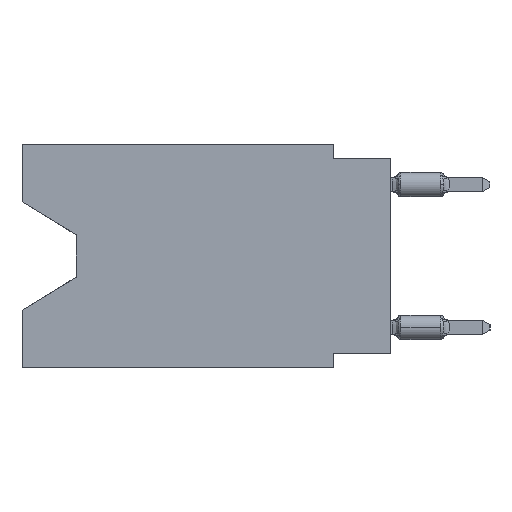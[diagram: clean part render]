
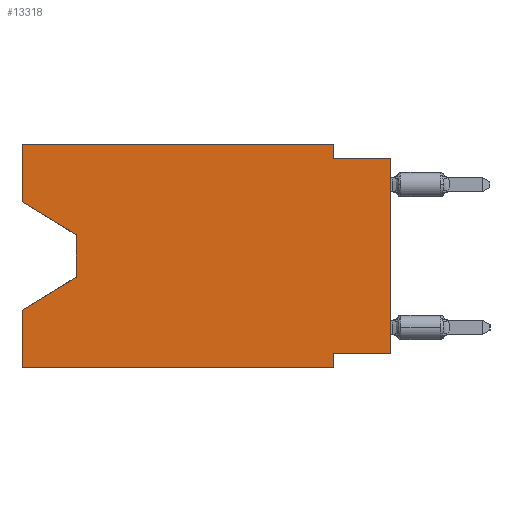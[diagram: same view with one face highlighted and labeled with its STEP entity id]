
A CAD part, left-side view. The second image highlights one B-rep face of the part: STEP entity #13318.
In plain terms, the highlighted planar face has unit normal (-1, 0, 0).
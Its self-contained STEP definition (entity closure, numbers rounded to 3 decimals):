
#568 = CARTESIAN_POINT ( 'NONE',  ( 0., 0., -9.271 ) ) ;
#723 = PLANE ( 'NONE',  #55464 ) ;
#1329 = VERTEX_POINT ( 'NONE', #13001 ) ;
#1730 = VERTEX_POINT ( 'NONE', #40131 ) ;
#1859 = DIRECTION ( 'NONE',  ( 0., 0.855, -0.519 ) ) ;
#2836 = VECTOR ( 'NONE', #10460, 1000. ) ;
#4807 = CARTESIAN_POINT ( 'NONE',  ( 0., 13.97, -5.893 ) ) ;
#6092 = DIRECTION ( 'NONE',  ( 0., 0., -1. ) ) ;
#6950 = LINE ( 'NONE', #62082, #31623 ) ;
#7746 = VERTEX_POINT ( 'NONE', #16965 ) ;
#8051 = VERTEX_POINT ( 'NONE', #4807 ) ;
#9061 = ORIENTED_EDGE ( 'NONE', *, *, #9385, .F. ) ;
#9385 = EDGE_CURVE ( 'NONE', #15146, #33059, #26433, .T. ) ;
#10120 = VERTEX_POINT ( 'NONE', #34221 ) ;
#10443 = EDGE_CURVE ( 'NONE', #60541, #45017, #34143, .T. ) ;
#10460 = DIRECTION ( 'NONE',  ( 0., 0., 1. ) ) ;
#10571 = EDGE_CURVE ( 'NONE', #13068, #45017, #55422, .T. ) ;
#11564 = ORIENTED_EDGE ( 'NONE', *, *, #10571, .T. ) ;
#13001 = CARTESIAN_POINT ( 'NONE',  ( 0., 16.383, 0. ) ) ;
#13068 = VERTEX_POINT ( 'NONE', #45047 ) ;
#13272 = EDGE_CURVE ( 'NONE', #7746, #8051, #41079, .T. ) ;
#13286 = ORIENTED_EDGE ( 'NONE', *, *, #41180, .T. ) ;
#13318 = ADVANCED_FACE ( 'NONE', ( #35832 ), #723, .F. ) ;
#14314 = VECTOR ( 'NONE', #6092, 1000. ) ;
#14420 = DIRECTION ( 'NONE',  ( 0., -1., 0. ) ) ;
#15146 = VERTEX_POINT ( 'NONE', #20239 ) ;
#16104 = EDGE_CURVE ( 'NONE', #53267, #1329, #44271, .T. ) ;
#16393 = DIRECTION ( 'NONE',  ( 0., -0.855, -0.519 ) ) ;
#16965 = CARTESIAN_POINT ( 'NONE',  ( 0., 13.97, -4.013 ) ) ;
#17095 = DIRECTION ( 'NONE',  ( 1., 0., 0. ) ) ;
#19294 = CARTESIAN_POINT ( 'NONE',  ( 0., 16.383, 0. ) ) ;
#19420 = CARTESIAN_POINT ( 'NONE',  ( 0., 2.54, -0.635 ) ) ;
#20239 = CARTESIAN_POINT ( 'NONE',  ( 0., 2.54, -9.271 ) ) ;
#20812 = EDGE_CURVE ( 'NONE', #1730, #60541, #23196, .T. ) ;
#20881 = LINE ( 'NONE', #568, #38752 ) ;
#20978 = VECTOR ( 'NONE', #16393, 1000. ) ;
#21396 = DIRECTION ( 'NONE',  ( 0., -1., 0. ) ) ;
#21693 = VECTOR ( 'NONE', #14420, 1000. ) ;
#23196 = LINE ( 'NONE', #32406, #49706 ) ;
#23734 = EDGE_CURVE ( 'NONE', #10120, #26596, #60609, .T. ) ;
#25001 = EDGE_CURVE ( 'NONE', #13068, #15146, #20881, .T. ) ;
#25100 = CARTESIAN_POINT ( 'NONE',  ( 0., 16.383, -9.906 ) ) ;
#26159 = ORIENTED_EDGE ( 'NONE', *, *, #42830, .F. ) ;
#26412 = EDGE_LOOP ( 'NONE', ( #13286, #37111, #46792, #61126, #58222, #9061, #44586, #11564, #39066, #61613, #26159, #39745 ) ) ;
#26433 = LINE ( 'NONE', #32013, #14314 ) ;
#26484 = CARTESIAN_POINT ( 'NONE',  ( 0., 16.383, -2.546 ) ) ;
#26596 = VERTEX_POINT ( 'NONE', #39900 ) ;
#29530 = VECTOR ( 'NONE', #35047, 1000. ) ;
#30913 = CARTESIAN_POINT ( 'NONE',  ( 0., 13.97, -4.013 ) ) ;
#31222 = DIRECTION ( 'NONE',  ( 0., 0., -1. ) ) ;
#31623 = VECTOR ( 'NONE', #21396, 1000. ) ;
#32001 = EDGE_CURVE ( 'NONE', #10120, #33059, #51000, .T. ) ;
#32013 = CARTESIAN_POINT ( 'NONE',  ( 0., 2.54, -9.906 ) ) ;
#32406 = CARTESIAN_POINT ( 'NONE',  ( 0., 2.54, 0. ) ) ;
#33059 = VERTEX_POINT ( 'NONE', #64493 ) ;
#33356 = LINE ( 'NONE', #53362, #51188 ) ;
#34143 = LINE ( 'NONE', #63008, #21693 ) ;
#34221 = CARTESIAN_POINT ( 'NONE',  ( 0., 16.383, -9.906 ) ) ;
#35047 = DIRECTION ( 'NONE',  ( 0., 0., 1. ) ) ;
#35345 = DIRECTION ( 'NONE',  ( 0., 0., 1. ) ) ;
#35832 = FACE_OUTER_BOUND ( 'NONE', #26412, .T. ) ;
#37111 = ORIENTED_EDGE ( 'NONE', *, *, #13272, .T. ) ;
#38304 = DIRECTION ( 'NONE',  ( 0., 0., -1. ) ) ;
#38752 = VECTOR ( 'NONE', #61895, 1000. ) ;
#39066 = ORIENTED_EDGE ( 'NONE', *, *, #10443, .F. ) ;
#39745 = ORIENTED_EDGE ( 'NONE', *, *, #16104, .F. ) ;
#39900 = CARTESIAN_POINT ( 'NONE',  ( 0., 16.383, -7.36 ) ) ;
#40131 = CARTESIAN_POINT ( 'NONE',  ( 0., 2.54, 0. ) ) ;
#40755 = DIRECTION ( 'NONE',  ( 0., 0., -1. ) ) ;
#41079 = LINE ( 'NONE', #30913, #46043 ) ;
#41180 = EDGE_CURVE ( 'NONE', #53267, #7746, #46616, .T. ) ;
#42830 = EDGE_CURVE ( 'NONE', #1329, #1730, #6950, .T. ) ;
#44271 = LINE ( 'NONE', #19294, #29530 ) ;
#44586 = ORIENTED_EDGE ( 'NONE', *, *, #25001, .F. ) ;
#45017 = VERTEX_POINT ( 'NONE', #62282 ) ;
#45047 = CARTESIAN_POINT ( 'NONE',  ( 0., 0., -9.271 ) ) ;
#45124 = DIRECTION ( 'NONE',  ( 0., -1., 0. ) ) ;
#45584 = CARTESIAN_POINT ( 'NONE',  ( 0., 0., 0. ) ) ;
#46043 = VECTOR ( 'NONE', #31222, 1000. ) ;
#46616 = LINE ( 'NONE', #56112, #20978 ) ;
#46792 = ORIENTED_EDGE ( 'NONE', *, *, #52120, .T. ) ;
#49706 = VECTOR ( 'NONE', #38304, 1000. ) ;
#51000 = LINE ( 'NONE', #25100, #62242 ) ;
#51188 = VECTOR ( 'NONE', #1859, 1000. ) ;
#52120 = EDGE_CURVE ( 'NONE', #8051, #26596, #33356, .T. ) ;
#53267 = VERTEX_POINT ( 'NONE', #26484 ) ;
#53362 = CARTESIAN_POINT ( 'NONE',  ( 0., 13.97, -5.893 ) ) ;
#55422 = LINE ( 'NONE', #45584, #2836 ) ;
#55464 = AXIS2_PLACEMENT_3D ( 'NONE', #60773, #17095, #40755 ) ;
#56112 = CARTESIAN_POINT ( 'NONE',  ( 0., 16.383, -2.546 ) ) ;
#58222 = ORIENTED_EDGE ( 'NONE', *, *, #32001, .T. ) ;
#60541 = VERTEX_POINT ( 'NONE', #19420 ) ;
#60609 = LINE ( 'NONE', #60915, #61672 ) ;
#60773 = CARTESIAN_POINT ( 'NONE',  ( 0., 16.383, 0. ) ) ;
#60915 = CARTESIAN_POINT ( 'NONE',  ( 0., 16.383, 0. ) ) ;
#61126 = ORIENTED_EDGE ( 'NONE', *, *, #23734, .F. ) ;
#61613 = ORIENTED_EDGE ( 'NONE', *, *, #20812, .F. ) ;
#61672 = VECTOR ( 'NONE', #35345, 1000. ) ;
#61895 = DIRECTION ( 'NONE',  ( 0., 1., 0. ) ) ;
#62082 = CARTESIAN_POINT ( 'NONE',  ( 0., 16.383, 0. ) ) ;
#62242 = VECTOR ( 'NONE', #45124, 1000. ) ;
#62282 = CARTESIAN_POINT ( 'NONE',  ( 0., 0., -0.635 ) ) ;
#63008 = CARTESIAN_POINT ( 'NONE',  ( 0., 0., -0.635 ) ) ;
#64493 = CARTESIAN_POINT ( 'NONE',  ( 0., 2.54, -9.906 ) ) ;
